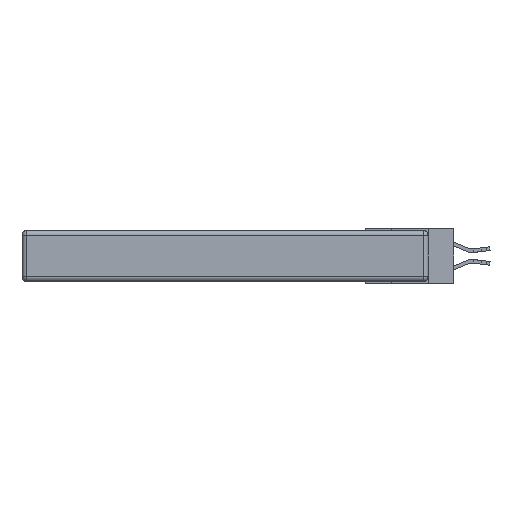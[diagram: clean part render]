
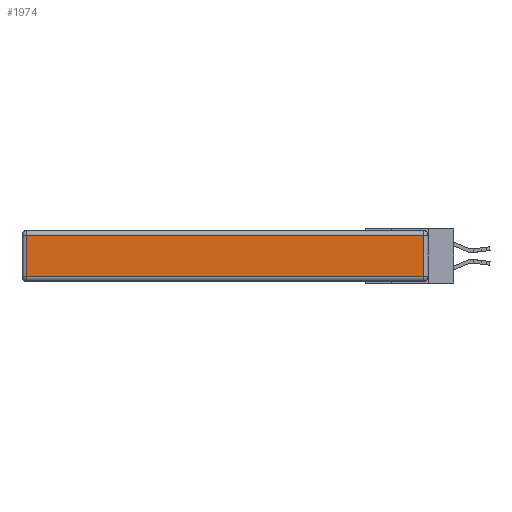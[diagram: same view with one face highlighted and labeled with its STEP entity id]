
A CAD part, left-side view. The second image highlights one B-rep face of the part: STEP entity #1974.
In plain terms, the highlighted planar face has unit normal (-1, 0, 0).
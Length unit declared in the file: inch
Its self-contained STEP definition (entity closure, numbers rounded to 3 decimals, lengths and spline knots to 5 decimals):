
#1232 = VECTOR ( 'NONE', #9640, 39.37008 ) ;
#1541 = CARTESIAN_POINT ( 'NONE',  ( 0., 0., -0.313 ) ) ;
#1731 = PLANE ( 'NONE',  #8246 ) ;
#1732 = CARTESIAN_POINT ( 'NONE',  ( 0., 2.72, -0.343 ) ) ;
#1974 = ADVANCED_FACE ( 'NONE', ( #15816 ), #1731, .T. ) ;
#2567 = VERTEX_POINT ( 'NONE', #5217 ) ;
#2881 = VERTEX_POINT ( 'NONE', #9172 ) ;
#2882 = EDGE_CURVE ( 'NONE', #2567, #8426, #13546, .T. ) ;
#3713 = CARTESIAN_POINT ( 'NONE',  ( 0., 0.03, -0.343 ) ) ;
#4371 = VECTOR ( 'NONE', #10119, 39.37008 ) ;
#5147 = LINE ( 'NONE', #1732, #1232 ) ;
#5217 = CARTESIAN_POINT ( 'NONE',  ( 0., 0.03, -0.03 ) ) ;
#6300 = VECTOR ( 'NONE', #8537, 39.37008 ) ;
#6516 = VECTOR ( 'NONE', #9116, 39.37008 ) ;
#7041 = VERTEX_POINT ( 'NONE', #9403 ) ;
#7797 = ORIENTED_EDGE ( 'NONE', *, *, #16143, .T. ) ;
#8246 = AXIS2_PLACEMENT_3D ( 'NONE', #8316, #11119, #9639 ) ;
#8316 = CARTESIAN_POINT ( 'NONE',  ( 0., 0., -0.343 ) ) ;
#8426 = VERTEX_POINT ( 'NONE', #12731 ) ;
#8537 = DIRECTION ( 'NONE',  ( 0., -1., 0. ) ) ;
#9116 = DIRECTION ( 'NONE',  ( 0., 1., 0. ) ) ;
#9172 = CARTESIAN_POINT ( 'NONE',  ( 0., 0.03, -0.313 ) ) ;
#9403 = CARTESIAN_POINT ( 'NONE',  ( 0., 2.72, -0.313 ) ) ;
#9639 = DIRECTION ( 'NONE',  ( 0., 0., 1. ) ) ;
#9640 = DIRECTION ( 'NONE',  ( 0., 0., -1. ) ) ;
#10119 = DIRECTION ( 'NONE',  ( 0., 0., 1. ) ) ;
#10559 = LINE ( 'NONE', #3713, #4371 ) ;
#11008 = EDGE_CURVE ( 'NONE', #7041, #2881, #12087, .T. ) ;
#11067 = ORIENTED_EDGE ( 'NONE', *, *, #12894, .T. ) ;
#11119 = DIRECTION ( 'NONE',  ( -1., 0., 0. ) ) ;
#11237 = ORIENTED_EDGE ( 'NONE', *, *, #2882, .T. ) ;
#12087 = LINE ( 'NONE', #1541, #6300 ) ;
#12731 = CARTESIAN_POINT ( 'NONE',  ( 0., 2.72, -0.03 ) ) ;
#12894 = EDGE_CURVE ( 'NONE', #2881, #2567, #10559, .T. ) ;
#13021 = CARTESIAN_POINT ( 'NONE',  ( 0., 2.75, -0.03 ) ) ;
#13546 = LINE ( 'NONE', #13021, #6516 ) ;
#14175 = EDGE_LOOP ( 'NONE', ( #15308, #11067, #11237, #7797 ) ) ;
#15308 = ORIENTED_EDGE ( 'NONE', *, *, #11008, .T. ) ;
#15816 = FACE_OUTER_BOUND ( 'NONE', #14175, .T. ) ;
#16143 = EDGE_CURVE ( 'NONE', #8426, #7041, #5147, .T. ) ;
